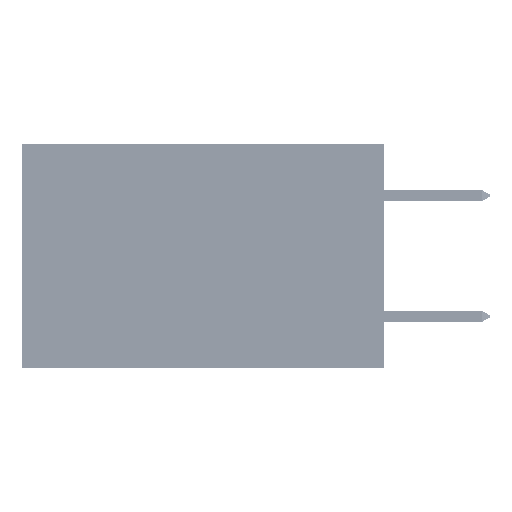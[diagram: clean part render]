
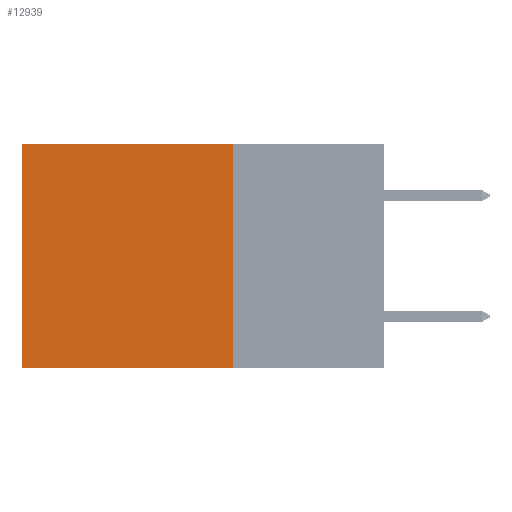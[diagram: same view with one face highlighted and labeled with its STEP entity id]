
A CAD part, left-side view. The second image highlights one B-rep face of the part: STEP entity #12939.
In plain terms, the highlighted planar face has unit normal (-1, 0, 0).
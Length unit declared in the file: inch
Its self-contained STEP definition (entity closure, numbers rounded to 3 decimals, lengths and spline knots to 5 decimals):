
#943 = EDGE_CURVE ( 'NONE', #29081, #37703, #21931, .T. ) ;
#3558 = EDGE_LOOP ( 'NONE', ( #50351, #37269, #8890, #26377 ) ) ;
#6493 = DIRECTION ( 'NONE',  ( 1., 0., 0. ) ) ;
#6580 = CARTESIAN_POINT ( 'NONE',  ( 0.2875, 0.6, 0. ) ) ;
#6846 = DIRECTION ( 'NONE',  ( 0., 0., -1. ) ) ;
#8890 = ORIENTED_EDGE ( 'NONE', *, *, #29178, .F. ) ;
#9995 = CARTESIAN_POINT ( 'NONE',  ( 0.2875, 0.25, -0.37 ) ) ;
#12939 = ADVANCED_FACE ( 'NONE', ( #25427 ), #30786, .F. ) ;
#16510 = CARTESIAN_POINT ( 'NONE',  ( 0.2875, 0.25, -0.37 ) ) ;
#16856 = DIRECTION ( 'NONE',  ( 0., 1., 0. ) ) ;
#17036 = CARTESIAN_POINT ( 'NONE',  ( 0.2875, 0.6, 0. ) ) ;
#17748 = LINE ( 'NONE', #26793, #26571 ) ;
#18911 = CARTESIAN_POINT ( 'NONE',  ( 0.2875, 0.25, 0. ) ) ;
#20063 = DIRECTION ( 'NONE',  ( 0., 0., -1. ) ) ;
#20091 = VECTOR ( 'NONE', #16856, 39.37008 ) ;
#21931 = LINE ( 'NONE', #16510, #20091 ) ;
#21962 = EDGE_CURVE ( 'NONE', #34761, #37703, #45675, .T. ) ;
#22873 = DIRECTION ( 'NONE',  ( 0., 0., -1. ) ) ;
#25427 = FACE_OUTER_BOUND ( 'NONE', #3558, .T. ) ;
#26052 = CARTESIAN_POINT ( 'NONE',  ( 0.2875, 0.6, -0.37 ) ) ;
#26377 = ORIENTED_EDGE ( 'NONE', *, *, #46952, .T. ) ;
#26571 = VECTOR ( 'NONE', #22873, 39.37008 ) ;
#26793 = CARTESIAN_POINT ( 'NONE',  ( 0.2875, 0.25, 0. ) ) ;
#29081 = VERTEX_POINT ( 'NONE', #9995 ) ;
#29178 = EDGE_CURVE ( 'NONE', #29716, #29081, #17748, .T. ) ;
#29716 = VERTEX_POINT ( 'NONE', #39752 ) ;
#30786 = PLANE ( 'NONE',  #41611 ) ;
#33843 = DIRECTION ( 'NONE',  ( 0., 1., 0. ) ) ;
#34189 = CARTESIAN_POINT ( 'NONE',  ( 0.2875, 0.25, 0. ) ) ;
#34761 = VERTEX_POINT ( 'NONE', #17036 ) ;
#36119 = VECTOR ( 'NONE', #20063, 39.37008 ) ;
#37269 = ORIENTED_EDGE ( 'NONE', *, *, #943, .F. ) ;
#37703 = VERTEX_POINT ( 'NONE', #26052 ) ;
#39752 = CARTESIAN_POINT ( 'NONE',  ( 0.2875, 0.25, 0. ) ) ;
#41611 = AXIS2_PLACEMENT_3D ( 'NONE', #18911, #6493, #6846 ) ;
#45675 = LINE ( 'NONE', #6580, #36119 ) ;
#46952 = EDGE_CURVE ( 'NONE', #29716, #34761, #51309, .T. ) ;
#50351 = ORIENTED_EDGE ( 'NONE', *, *, #21962, .T. ) ;
#51309 = LINE ( 'NONE', #34189, #52581 ) ;
#52581 = VECTOR ( 'NONE', #33843, 39.37008 ) ;
